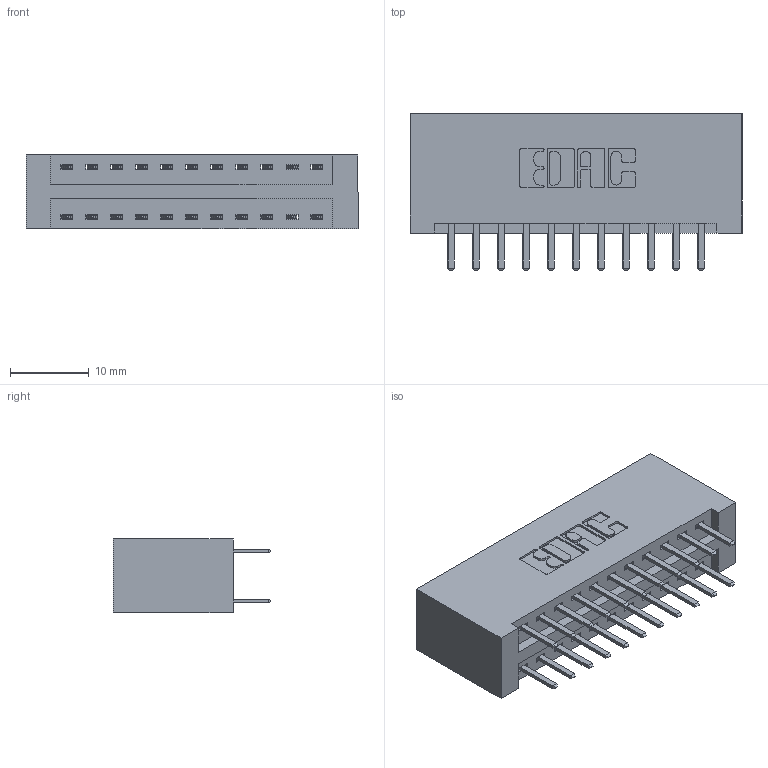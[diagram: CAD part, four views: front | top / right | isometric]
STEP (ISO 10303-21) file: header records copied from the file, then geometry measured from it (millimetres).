
FILE_DESCRIPTION (( 'STEP AP203' ), '1' );
FILE_NAME ('346-022-520-201.STEP', '2022-05-18T20:34:17', ( '' ), ( '' ), 'SwSTEP 2.0', 'SolidWorks 2020', '' );
FILE_SCHEMA (( 'CONFIG_CONTROL_DESIGN' ));
Length unit declared in the file: inch
Products named in the file (3): 346 Part_No Mounting Lugs; 346-022-520-201; 345-292-001_345-293-120
Assembly tree (23 placements, depth 2):
  346-022-520-201
    346 Part_No Mounting Lugs
    345-292-001_345-293-120  x22
Bounding box: 42.16 x 20.02 x 9.4 mm (x, y, z)
Volume: 4434.4 mm3; surface area: 5748.6 mm2
Topology: 23 solids, 23 shells, 1346 faces, 3891 edges, 2534 vertices
Faces by surface type: plane 886, cylinder 460
Entity records: 11189 total; most frequent: CARTESIAN_POINT 1896, ORIENTED_EDGE 1818, DIRECTION 1705, EDGE_CURVE 909, VECTOR 737, LINE 737, VERTEX_POINT 602, AXIS2_PLACEMENT_3D 484
